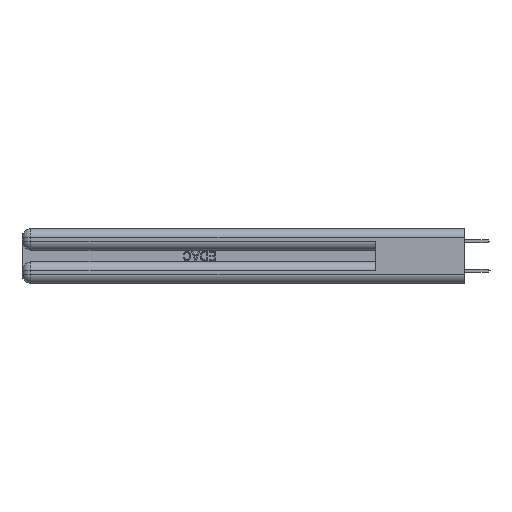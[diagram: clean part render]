
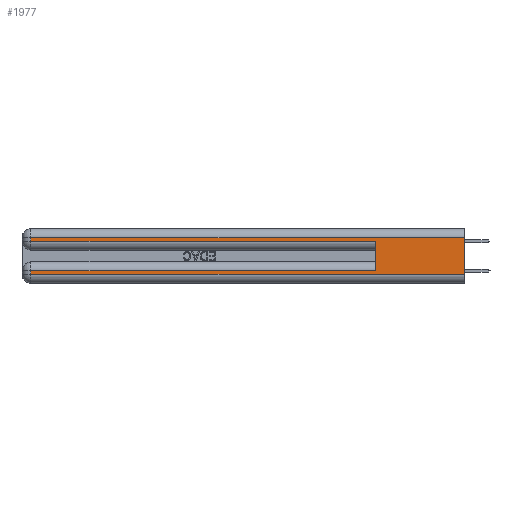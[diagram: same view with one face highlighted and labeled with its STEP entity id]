
A CAD part, left-side view. The second image highlights one B-rep face of the part: STEP entity #1977.
In plain terms, the highlighted planar face has unit normal (-1, 0, 0).
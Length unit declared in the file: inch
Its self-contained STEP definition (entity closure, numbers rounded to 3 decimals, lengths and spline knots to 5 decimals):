
#491 = VERTEX_POINT ( 'NONE', #7829 ) ;
#626 = VERTEX_POINT ( 'NONE', #26955 ) ;
#1664 = LINE ( 'NONE', #29959, #7896 ) ;
#1977 = ADVANCED_FACE ( 'NONE', ( #36711 ), #4857, .F. ) ;
#1982 = CARTESIAN_POINT ( 'NONE',  ( 0., 0.6, 0.285 ) ) ;
#3397 = ORIENTED_EDGE ( 'NONE', *, *, #36591, .T. ) ;
#4011 = DIRECTION ( 'NONE',  ( 0., 0., -1. ) ) ;
#4857 = PLANE ( 'NONE',  #15479 ) ;
#7829 = CARTESIAN_POINT ( 'NONE',  ( 0., 0., 0.06 ) ) ;
#7896 = VECTOR ( 'NONE', #26004, 39.37008 ) ;
#9720 = CARTESIAN_POINT ( 'NONE',  ( 0., 0., 0.31 ) ) ;
#13399 = CARTESIAN_POINT ( 'NONE',  ( 0., 2.94, 0.06 ) ) ;
#13796 = LINE ( 'NONE', #34919, #14937 ) ;
#14179 = ORIENTED_EDGE ( 'NONE', *, *, #26221, .T. ) ;
#14937 = VECTOR ( 'NONE', #42321, 39.37008 ) ;
#15479 = AXIS2_PLACEMENT_3D ( 'NONE', #23140, #19677, #34851 ) ;
#16375 = ORIENTED_EDGE ( 'NONE', *, *, #45665, .T. ) ;
#16482 = CARTESIAN_POINT ( 'NONE',  ( 0., 0.6, 0.145 ) ) ;
#16539 = VECTOR ( 'NONE', #31519, 39.37008 ) ;
#17449 = VERTEX_POINT ( 'NONE', #1982 ) ;
#17454 = DIRECTION ( 'NONE',  ( 0., -1., 0. ) ) ;
#18205 = CARTESIAN_POINT ( 'NONE',  ( 0., 0., 0.37 ) ) ;
#19677 = DIRECTION ( 'NONE',  ( 1., 0., 0. ) ) ;
#19945 = VECTOR ( 'NONE', #29439, 39.37008 ) ;
#20550 = ORIENTED_EDGE ( 'NONE', *, *, #30312, .T. ) ;
#22199 = VECTOR ( 'NONE', #41688, 39.37008 ) ;
#22922 = CARTESIAN_POINT ( 'NONE',  ( 0., 2.94, 0.31 ) ) ;
#22961 = LINE ( 'NONE', #9720, #31470 ) ;
#23140 = CARTESIAN_POINT ( 'NONE',  ( 0., 0., 0.37 ) ) ;
#24024 = ORIENTED_EDGE ( 'NONE', *, *, #37252, .F. ) ;
#24109 = ORIENTED_EDGE ( 'NONE', *, *, #28451, .T. ) ;
#24955 = LINE ( 'NONE', #26844, #22199 ) ;
#25713 = CARTESIAN_POINT ( 'NONE',  ( 0., 2.94, 0.285 ) ) ;
#26004 = DIRECTION ( 'NONE',  ( 0., 1., 0. ) ) ;
#26162 = LINE ( 'NONE', #18205, #19945 ) ;
#26221 = EDGE_CURVE ( 'NONE', #626, #40310, #1664, .T. ) ;
#26844 = CARTESIAN_POINT ( 'NONE',  ( 0., 2.94, 0.37 ) ) ;
#26955 = CARTESIAN_POINT ( 'NONE',  ( 0., 0.6, 0.085 ) ) ;
#28451 = EDGE_CURVE ( 'NONE', #37913, #40995, #22961, .T. ) ;
#29439 = DIRECTION ( 'NONE',  ( 0., 0., -1. ) ) ;
#29959 = CARTESIAN_POINT ( 'NONE',  ( 0., 0., 0.085 ) ) ;
#30312 = EDGE_CURVE ( 'NONE', #40310, #45692, #42318, .T. ) ;
#31470 = VECTOR ( 'NONE', #46451, 39.37008 ) ;
#31519 = DIRECTION ( 'NONE',  ( 0., 0., 1. ) ) ;
#32085 = VECTOR ( 'NONE', #17454, 39.37008 ) ;
#32715 = VECTOR ( 'NONE', #4011, 39.37008 ) ;
#33631 = EDGE_CURVE ( 'NONE', #37913, #491, #26162, .T. ) ;
#34851 = DIRECTION ( 'NONE',  ( 0., 0., -1. ) ) ;
#34919 = CARTESIAN_POINT ( 'NONE',  ( 0., 0., 0.06 ) ) ;
#36591 = EDGE_CURVE ( 'NONE', #40995, #39417, #24955, .T. ) ;
#36711 = FACE_OUTER_BOUND ( 'NONE', #37863, .T. ) ;
#37252 = EDGE_CURVE ( 'NONE', #626, #17449, #43632, .T. ) ;
#37863 = EDGE_LOOP ( 'NONE', ( #45347, #24109, #3397, #40638, #24024, #14179, #20550, #16375 ) ) ;
#37913 = VERTEX_POINT ( 'NONE', #45320 ) ;
#39110 = CARTESIAN_POINT ( 'NONE',  ( 0., 0., 0.285 ) ) ;
#39417 = VERTEX_POINT ( 'NONE', #25713 ) ;
#40032 = EDGE_CURVE ( 'NONE', #39417, #17449, #46145, .T. ) ;
#40310 = VERTEX_POINT ( 'NONE', #41279 ) ;
#40532 = CARTESIAN_POINT ( 'NONE',  ( 0., 2.94, 0.37 ) ) ;
#40638 = ORIENTED_EDGE ( 'NONE', *, *, #40032, .T. ) ;
#40995 = VERTEX_POINT ( 'NONE', #22922 ) ;
#41279 = CARTESIAN_POINT ( 'NONE',  ( 0., 2.94, 0.085 ) ) ;
#41688 = DIRECTION ( 'NONE',  ( 0., 0., -1. ) ) ;
#42318 = LINE ( 'NONE', #40532, #32715 ) ;
#42321 = DIRECTION ( 'NONE',  ( 0., -1., 0. ) ) ;
#43632 = LINE ( 'NONE', #16482, #16539 ) ;
#45320 = CARTESIAN_POINT ( 'NONE',  ( 0., 0., 0.31 ) ) ;
#45347 = ORIENTED_EDGE ( 'NONE', *, *, #33631, .F. ) ;
#45665 = EDGE_CURVE ( 'NONE', #45692, #491, #13796, .T. ) ;
#45692 = VERTEX_POINT ( 'NONE', #13399 ) ;
#46145 = LINE ( 'NONE', #39110, #32085 ) ;
#46451 = DIRECTION ( 'NONE',  ( 0., 1., 0. ) ) ;
